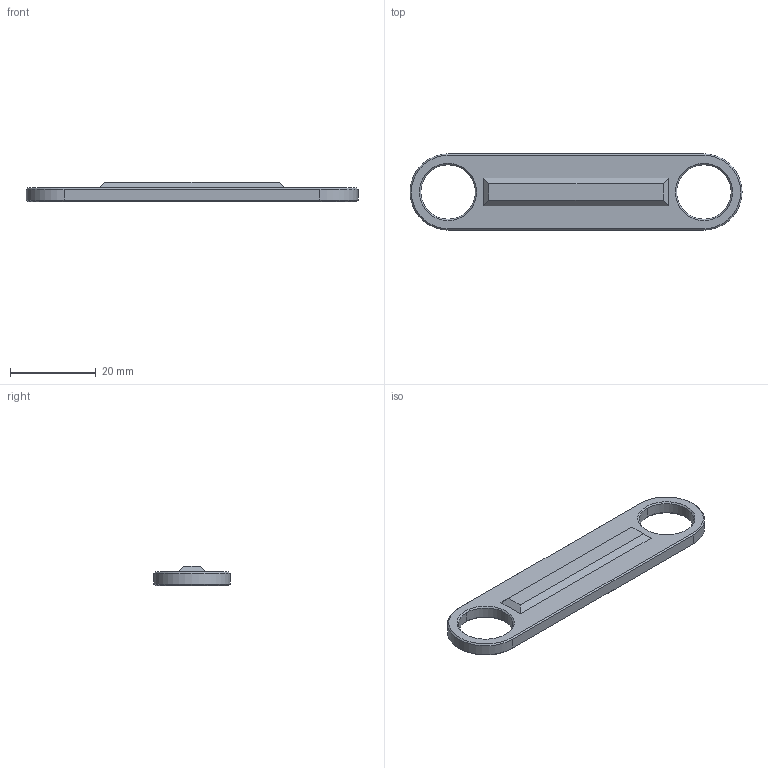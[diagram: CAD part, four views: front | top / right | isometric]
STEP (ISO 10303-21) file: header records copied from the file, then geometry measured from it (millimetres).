
FILE_DESCRIPTION (( 'STEP AP203' ), '1' );
FILE_NAME ('AF-GFP-MP-PRT-002-STEP.STEP', '2020-08-04T07:32:26', ( '' ), ( '' ), 'SwSTEP 2.0', 'SolidWorks 2018', '' );
FILE_SCHEMA (( 'CONFIG_CONTROL_DESIGN' ));
Length unit declared in the file: inch
Products named in the file (1): AF-GFP-MP-PRT-002-STEP
Bounding box: 77.47 x 17.78 x 4.45 mm (x, y, z)
Volume: 3590.3 mm3; surface area: 2932.5 mm2
Topology: 1 solids, 1 shells, 224 faces, 575 edges, 378 vertices
Faces by surface type: plane 150, bspline 56, cone 12, cylinder 6
Entity records: 10470 total; most frequent: CARTESIAN_POINT 5298, ORIENTED_EDGE 1150, DIRECTION 825, EDGE_CURVE 575, LINE 439, VECTOR 439, VERTEX_POINT 378, EDGE_LOOP 253
